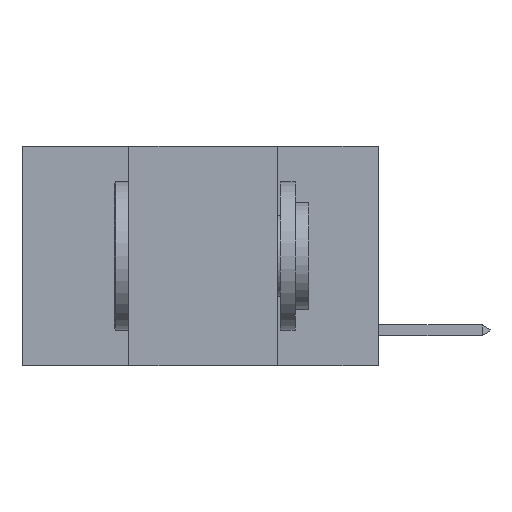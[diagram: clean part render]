
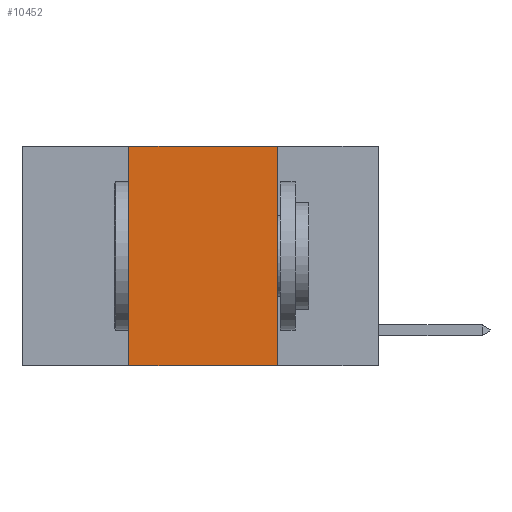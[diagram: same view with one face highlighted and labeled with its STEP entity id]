
A CAD part, left-side view. The second image highlights one B-rep face of the part: STEP entity #10452.
In plain terms, the highlighted planar face has unit normal (-1, 0, 0).
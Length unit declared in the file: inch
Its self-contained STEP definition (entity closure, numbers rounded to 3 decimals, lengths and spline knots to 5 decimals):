
#317 = VERTEX_POINT ( 'NONE', #2774 ) ;
#1060 = FACE_OUTER_BOUND ( 'NONE', #12671, .T. ) ;
#1390 = EDGE_CURVE ( 'NONE', #11945, #7337, #7665, .T. ) ;
#1767 = ORIENTED_EDGE ( 'NONE', *, *, #1390, .F. ) ;
#1804 = VECTOR ( 'NONE', #10130, 39.37008 ) ;
#2117 = CARTESIAN_POINT ( 'NONE',  ( 0., 0.42, 0. ) ) ;
#2774 = CARTESIAN_POINT ( 'NONE',  ( 0., 0.17, -0.37 ) ) ;
#2802 = VERTEX_POINT ( 'NONE', #12703 ) ;
#2925 = AXIS2_PLACEMENT_3D ( 'NONE', #9063, #8188, #12275 ) ;
#4161 = CARTESIAN_POINT ( 'NONE',  ( 0., 0.6, -0.37 ) ) ;
#4655 = EDGE_CURVE ( 'NONE', #7337, #2802, #12213, .T. ) ;
#4864 = LINE ( 'NONE', #4936, #5057 ) ;
#4936 = CARTESIAN_POINT ( 'NONE',  ( 0., 0.17, 0. ) ) ;
#5028 = CARTESIAN_POINT ( 'NONE',  ( 0., 0.6, 0. ) ) ;
#5057 = VECTOR ( 'NONE', #8959, 39.37008 ) ;
#5307 = VECTOR ( 'NONE', #8262, 39.37008 ) ;
#6850 = ORIENTED_EDGE ( 'NONE', *, *, #11840, .T. ) ;
#7053 = PLANE ( 'NONE',  #2925 ) ;
#7337 = VERTEX_POINT ( 'NONE', #2117 ) ;
#7441 = CARTESIAN_POINT ( 'NONE',  ( 0., 0.42, -0.37 ) ) ;
#7665 = LINE ( 'NONE', #8624, #13102 ) ;
#8188 = DIRECTION ( 'NONE',  ( 1., 0., 0. ) ) ;
#8262 = DIRECTION ( 'NONE',  ( 0., -1., 0. ) ) ;
#8624 = CARTESIAN_POINT ( 'NONE',  ( 0., 0.42, 0. ) ) ;
#8771 = EDGE_CURVE ( 'NONE', #2802, #317, #4864, .T. ) ;
#8959 = DIRECTION ( 'NONE',  ( 0., 0., -1. ) ) ;
#9063 = CARTESIAN_POINT ( 'NONE',  ( 0., 0.6, 0. ) ) ;
#10130 = DIRECTION ( 'NONE',  ( 0., -1., 0. ) ) ;
#10179 = ORIENTED_EDGE ( 'NONE', *, *, #8771, .F. ) ;
#10271 = LINE ( 'NONE', #4161, #5307 ) ;
#10452 = ADVANCED_FACE ( 'NONE', ( #1060 ), #7053, .F. ) ;
#10638 = ORIENTED_EDGE ( 'NONE', *, *, #4655, .F. ) ;
#10826 = DIRECTION ( 'NONE',  ( 0., 0., 1. ) ) ;
#11840 = EDGE_CURVE ( 'NONE', #11945, #317, #10271, .T. ) ;
#11945 = VERTEX_POINT ( 'NONE', #7441 ) ;
#12213 = LINE ( 'NONE', #5028, #1804 ) ;
#12275 = DIRECTION ( 'NONE',  ( 0., 0., -1. ) ) ;
#12671 = EDGE_LOOP ( 'NONE', ( #10179, #10638, #1767, #6850 ) ) ;
#12703 = CARTESIAN_POINT ( 'NONE',  ( 0., 0.17, 0. ) ) ;
#13102 = VECTOR ( 'NONE', #10826, 39.37008 ) ;
